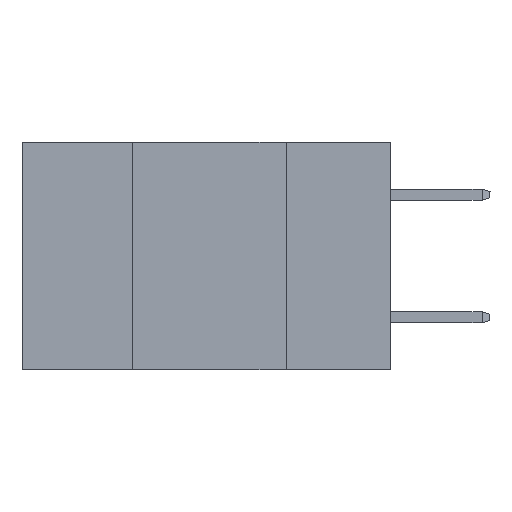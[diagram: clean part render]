
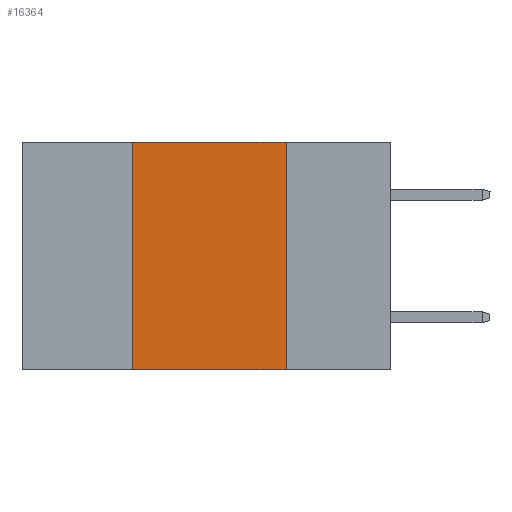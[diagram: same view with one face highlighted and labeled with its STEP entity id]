
A CAD part, left-side view. The second image highlights one B-rep face of the part: STEP entity #16364.
In plain terms, the highlighted planar face has unit normal (-1, 0, 0).
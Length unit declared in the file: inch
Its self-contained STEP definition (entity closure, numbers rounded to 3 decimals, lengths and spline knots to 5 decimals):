
#28 = VECTOR ( 'NONE', #26313, 39.37008 ) ;
#2593 = VECTOR ( 'NONE', #20217, 39.37008 ) ;
#2599 = LINE ( 'NONE', #14217, #28 ) ;
#3132 = CARTESIAN_POINT ( 'NONE',  ( 0., 0.42, -0.37 ) ) ;
#3174 = VERTEX_POINT ( 'NONE', #26176 ) ;
#3977 = CARTESIAN_POINT ( 'NONE',  ( 0., 0.6, -0.37 ) ) ;
#4161 = DIRECTION ( 'NONE',  ( 0., 0., -1. ) ) ;
#4233 = VERTEX_POINT ( 'NONE', #3132 ) ;
#4648 = EDGE_CURVE ( 'NONE', #4233, #13906, #2599, .T. ) ;
#4890 = EDGE_LOOP ( 'NONE', ( #15885, #15195, #5388, #14764 ) ) ;
#5388 = ORIENTED_EDGE ( 'NONE', *, *, #4648, .F. ) ;
#6041 = DIRECTION ( 'NONE',  ( 0., -1., 0. ) ) ;
#6659 = CARTESIAN_POINT ( 'NONE',  ( 0., 0.17, 0. ) ) ;
#8218 = VECTOR ( 'NONE', #23204, 39.37008 ) ;
#8229 = EDGE_CURVE ( 'NONE', #4233, #13217, #15104, .T. ) ;
#9804 = CARTESIAN_POINT ( 'NONE',  ( 0., 0.6, 0. ) ) ;
#10074 = FACE_OUTER_BOUND ( 'NONE', #4890, .T. ) ;
#10937 = EDGE_CURVE ( 'NONE', #3174, #13217, #26180, .T. ) ;
#11322 = EDGE_CURVE ( 'NONE', #13906, #3174, #17213, .T. ) ;
#13217 = VERTEX_POINT ( 'NONE', #22239 ) ;
#13906 = VERTEX_POINT ( 'NONE', #23241 ) ;
#14217 = CARTESIAN_POINT ( 'NONE',  ( 0., 0.42, 0. ) ) ;
#14764 = ORIENTED_EDGE ( 'NONE', *, *, #8229, .T. ) ;
#14963 = VECTOR ( 'NONE', #6041, 39.37008 ) ;
#15104 = LINE ( 'NONE', #3977, #2593 ) ;
#15195 = ORIENTED_EDGE ( 'NONE', *, *, #11322, .F. ) ;
#15885 = ORIENTED_EDGE ( 'NONE', *, *, #10937, .F. ) ;
#16364 = ADVANCED_FACE ( 'NONE', ( #10074 ), #22359, .F. ) ;
#16459 = CARTESIAN_POINT ( 'NONE',  ( 0., 0.6, 0. ) ) ;
#17213 = LINE ( 'NONE', #9804, #14963 ) ;
#18879 = DIRECTION ( 'NONE',  ( 1., 0., 0. ) ) ;
#20217 = DIRECTION ( 'NONE',  ( 0., -1., 0. ) ) ;
#22239 = CARTESIAN_POINT ( 'NONE',  ( 0., 0.17, -0.37 ) ) ;
#22359 = PLANE ( 'NONE',  #26224 ) ;
#23204 = DIRECTION ( 'NONE',  ( 0., 0., -1. ) ) ;
#23241 = CARTESIAN_POINT ( 'NONE',  ( 0., 0.42, 0. ) ) ;
#26176 = CARTESIAN_POINT ( 'NONE',  ( 0., 0.17, 0. ) ) ;
#26180 = LINE ( 'NONE', #6659, #8218 ) ;
#26224 = AXIS2_PLACEMENT_3D ( 'NONE', #16459, #18879, #4161 ) ;
#26313 = DIRECTION ( 'NONE',  ( 0., 0., 1. ) ) ;
